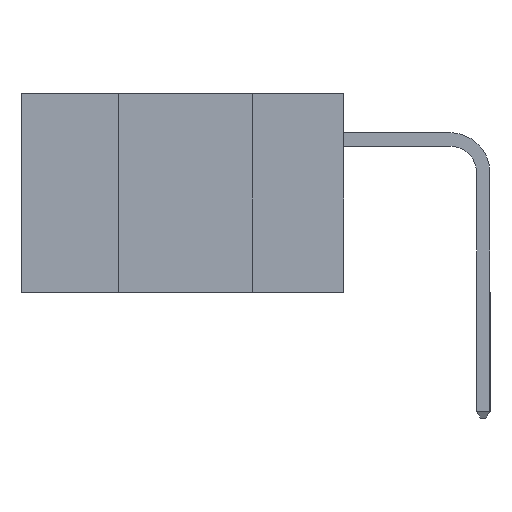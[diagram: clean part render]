
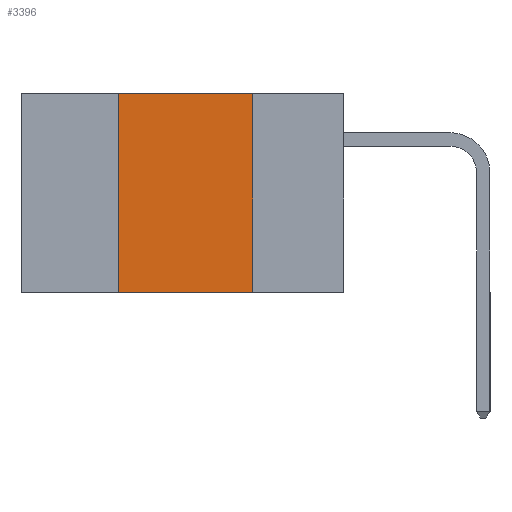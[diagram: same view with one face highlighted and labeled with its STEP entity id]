
A CAD part, left-side view. The second image highlights one B-rep face of the part: STEP entity #3396.
In plain terms, the highlighted planar face has unit normal (-1, 0, 0).
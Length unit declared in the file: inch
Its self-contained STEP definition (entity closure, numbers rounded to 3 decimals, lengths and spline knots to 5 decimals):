
#156 = EDGE_CURVE ( 'NONE', #8432, #14433, #12270, .T. ) ;
#514 = ORIENTED_EDGE ( 'NONE', *, *, #5974, .F. ) ;
#607 = ORIENTED_EDGE ( 'NONE', *, *, #10914, .F. ) ;
#811 = ORIENTED_EDGE ( 'NONE', *, *, #156, .T. ) ;
#1651 = ORIENTED_EDGE ( 'NONE', *, *, #12106, .F. ) ;
#1961 = VECTOR ( 'NONE', #11321, 39.37008 ) ;
#2312 = LINE ( 'NONE', #7811, #19901 ) ;
#2548 = VECTOR ( 'NONE', #20882, 39.37008 ) ;
#2808 = DIRECTION ( 'NONE',  ( 1., 0., 0. ) ) ;
#3396 = ADVANCED_FACE ( 'NONE', ( #10414 ), #21441, .F. ) ;
#3753 = DIRECTION ( 'NONE',  ( 0., 0., -1. ) ) ;
#4286 = CARTESIAN_POINT ( 'NONE',  ( 0., 0.6, 0. ) ) ;
#5974 = EDGE_CURVE ( 'NONE', #7921, #12306, #15844, .T. ) ;
#7811 = CARTESIAN_POINT ( 'NONE',  ( 0., 0.42, 0. ) ) ;
#7921 = VERTEX_POINT ( 'NONE', #17243 ) ;
#8432 = VERTEX_POINT ( 'NONE', #11989 ) ;
#9790 = CARTESIAN_POINT ( 'NONE',  ( 0., 0.17, 0. ) ) ;
#10414 = FACE_OUTER_BOUND ( 'NONE', #19755, .T. ) ;
#10832 = LINE ( 'NONE', #14373, #2548 ) ;
#10914 = EDGE_CURVE ( 'NONE', #8432, #7921, #2312, .T. ) ;
#11321 = DIRECTION ( 'NONE',  ( 0., -1., 0. ) ) ;
#11989 = CARTESIAN_POINT ( 'NONE',  ( 0., 0.42, -0.37 ) ) ;
#12106 = EDGE_CURVE ( 'NONE', #12306, #14433, #10832, .T. ) ;
#12270 = LINE ( 'NONE', #17110, #20950 ) ;
#12306 = VERTEX_POINT ( 'NONE', #9790 ) ;
#14373 = CARTESIAN_POINT ( 'NONE',  ( 0., 0.17, 0. ) ) ;
#14433 = VERTEX_POINT ( 'NONE', #21166 ) ;
#15844 = LINE ( 'NONE', #4286, #1961 ) ;
#17110 = CARTESIAN_POINT ( 'NONE',  ( 0., 0.6, -0.37 ) ) ;
#17243 = CARTESIAN_POINT ( 'NONE',  ( 0., 0.42, 0. ) ) ;
#17576 = DIRECTION ( 'NONE',  ( 0., -1., 0. ) ) ;
#18003 = CARTESIAN_POINT ( 'NONE',  ( 0., 0.6, 0. ) ) ;
#19550 = DIRECTION ( 'NONE',  ( 0., 0., 1. ) ) ;
#19755 = EDGE_LOOP ( 'NONE', ( #1651, #514, #607, #811 ) ) ;
#19901 = VECTOR ( 'NONE', #19550, 39.37008 ) ;
#20882 = DIRECTION ( 'NONE',  ( 0., 0., -1. ) ) ;
#20950 = VECTOR ( 'NONE', #17576, 39.37008 ) ;
#21166 = CARTESIAN_POINT ( 'NONE',  ( 0., 0.17, -0.37 ) ) ;
#21441 = PLANE ( 'NONE',  #22024 ) ;
#22024 = AXIS2_PLACEMENT_3D ( 'NONE', #18003, #2808, #3753 ) ;
